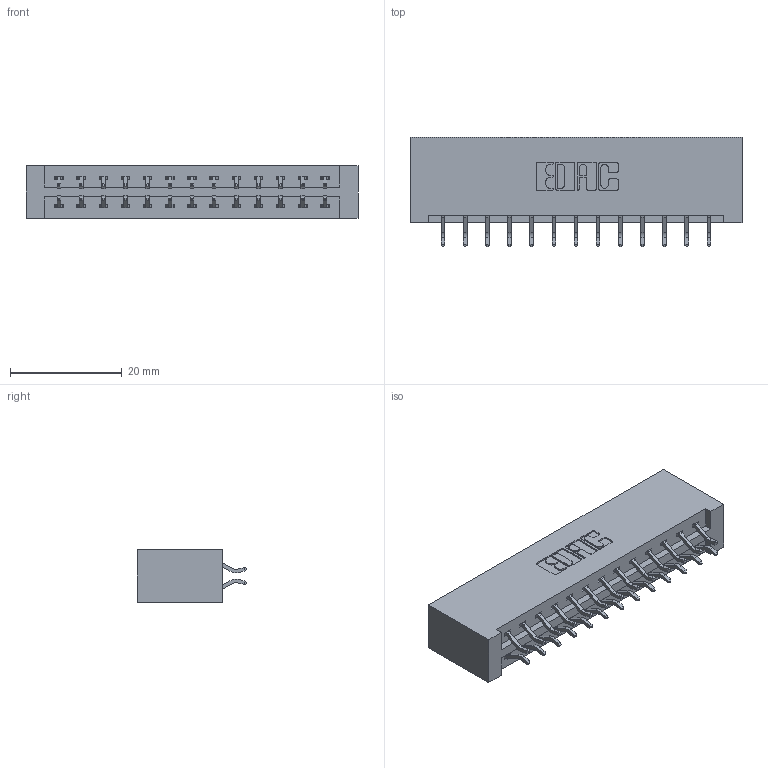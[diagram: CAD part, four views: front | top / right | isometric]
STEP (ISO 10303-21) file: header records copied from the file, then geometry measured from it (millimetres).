
FILE_DESCRIPTION (( 'STEP AP203' ), '1' );
FILE_NAME ('387-026-556-201.STEP', '2018-09-16T08:58:08', ( '' ), ( '' ), 'SwSTEP 2.0', 'SolidWorks 2016', '' );
FILE_SCHEMA (( 'CONFIG_CONTROL_DESIGN' ));
Length unit declared in the file: inch
Products named in the file (3): 337 Part_No Mounting Lugs; 345-292-001_556 Tail; 387-026-556-201
Assembly tree (27 placements, depth 2):
  387-026-556-201
    337 Part_No Mounting Lugs
    345-292-001_556 Tail  x26
Bounding box: 59.39 x 19.57 x 9.4 mm (x, y, z)
Volume: 6632.2 mm3; surface area: 7244.7 mm2
Topology: 27 solids, 27 shells, 1666 faces, 4941 edges, 3258 vertices
Faces by surface type: plane 1158, cylinder 508
Entity records: 13773 total; most frequent: CARTESIAN_POINT 2358, ORIENTED_EDGE 2282, DIRECTION 2041, EDGE_CURVE 1141, LINE 1013, VECTOR 1013, VERTEX_POINT 758, AXIS2_PLACEMENT_3D 514
